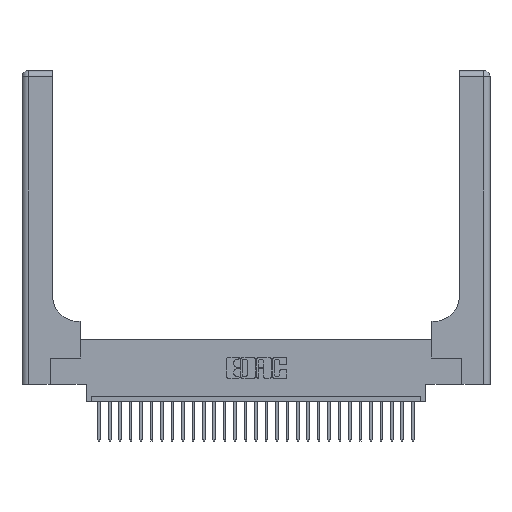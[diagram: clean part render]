
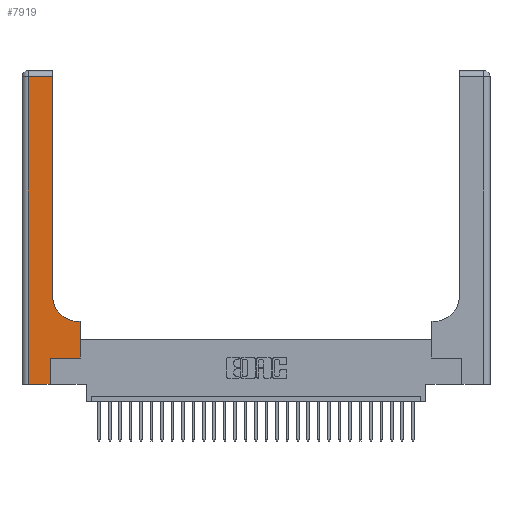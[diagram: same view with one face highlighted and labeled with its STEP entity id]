
A CAD part, top view. The second image highlights one B-rep face of the part: STEP entity #7919.
In plain terms, the highlighted planar face has unit normal (0, 0, 1).
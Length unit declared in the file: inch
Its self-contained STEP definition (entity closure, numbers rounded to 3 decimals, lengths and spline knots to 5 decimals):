
#313 = VECTOR ( 'NONE', #22695, 39.37008 ) ;
#1275 = LINE ( 'NONE', #13451, #19869 ) ;
#1321 = VERTEX_POINT ( 'NONE', #15081 ) ;
#1476 = VECTOR ( 'NONE', #20335, 39.37008 ) ;
#2177 = VERTEX_POINT ( 'NONE', #14005 ) ;
#2541 = VECTOR ( 'NONE', #29848, 39.37008 ) ;
#3033 = VERTEX_POINT ( 'NONE', #15591 ) ;
#3550 = LINE ( 'NONE', #24825, #9059 ) ;
#4838 = FACE_OUTER_BOUND ( 'NONE', #28960, .T. ) ;
#5357 = VERTEX_POINT ( 'NONE', #7960 ) ;
#5695 = CIRCLE ( 'NONE', #26918, 0.25 ) ;
#5790 = VECTOR ( 'NONE', #11148, 39.37008 ) ;
#6203 = VERTEX_POINT ( 'NONE', #27442 ) ;
#6899 = CARTESIAN_POINT ( 'NONE',  ( 0.5415, 0.85, 0.37 ) ) ;
#7050 = ORIENTED_EDGE ( 'NONE', *, *, #10753, .T. ) ;
#7227 = LINE ( 'NONE', #27291, #313 ) ;
#7815 = LINE ( 'NONE', #10754, #18358 ) ;
#7863 = DIRECTION ( 'NONE',  ( -1., 0., 0. ) ) ;
#7919 = ADVANCED_FACE ( 'NONE', ( #4838 ), #24490, .F. ) ;
#7934 = CARTESIAN_POINT ( 'NONE',  ( 0.269, 0.25, 0.37 ) ) ;
#7960 = CARTESIAN_POINT ( 'NONE',  ( 0.5585, 0.6, 0.37 ) ) ;
#8285 = CARTESIAN_POINT ( 'NONE',  ( 0., 3., 0.37 ) ) ;
#8692 = CARTESIAN_POINT ( 'NONE',  ( 0.06, 2.94, 0.37 ) ) ;
#9059 = VECTOR ( 'NONE', #10850, 39.37008 ) ;
#10523 = DIRECTION ( 'NONE',  ( 0., 0., -1. ) ) ;
#10753 = EDGE_CURVE ( 'NONE', #6203, #20432, #12018, .T. ) ;
#10754 = CARTESIAN_POINT ( 'NONE',  ( 0.2915, 0.6, 0.37 ) ) ;
#10850 = DIRECTION ( 'NONE',  ( 1., 0., 0. ) ) ;
#11148 = DIRECTION ( 'NONE',  ( -1., 0., 0. ) ) ;
#11509 = DIRECTION ( 'NONE',  ( 1., 0., 0. ) ) ;
#12018 = LINE ( 'NONE', #15990, #5790 ) ;
#12317 = EDGE_CURVE ( 'NONE', #16109, #14311, #1275, .T. ) ;
#12753 = ORIENTED_EDGE ( 'NONE', *, *, #21184, .T. ) ;
#13207 = CARTESIAN_POINT ( 'NONE',  ( 0.2915, 3., 0.37 ) ) ;
#13451 = CARTESIAN_POINT ( 'NONE',  ( 0.269, 0., 0.37 ) ) ;
#13736 = ORIENTED_EDGE ( 'NONE', *, *, #22083, .T. ) ;
#14005 = CARTESIAN_POINT ( 'NONE',  ( 0.5585, 0.25, 0.37 ) ) ;
#14012 = ORIENTED_EDGE ( 'NONE', *, *, #25195, .T. ) ;
#14311 = VERTEX_POINT ( 'NONE', #7934 ) ;
#14428 = ORIENTED_EDGE ( 'NONE', *, *, #27021, .T. ) ;
#15081 = CARTESIAN_POINT ( 'NONE',  ( 0.2915, 0.85, 0.37 ) ) ;
#15227 = ORIENTED_EDGE ( 'NONE', *, *, #12317, .T. ) ;
#15591 = CARTESIAN_POINT ( 'NONE',  ( 0.5415, 0.6, 0.37 ) ) ;
#15620 = ORIENTED_EDGE ( 'NONE', *, *, #22857, .T. ) ;
#15990 = CARTESIAN_POINT ( 'NONE',  ( 0., 2.94, 0.37 ) ) ;
#16078 = CARTESIAN_POINT ( 'NONE',  ( 0., 0., 0.37 ) ) ;
#16109 = VERTEX_POINT ( 'NONE', #17116 ) ;
#16749 = LINE ( 'NONE', #16078, #2541 ) ;
#17116 = CARTESIAN_POINT ( 'NONE',  ( 0.269, 0., 0.37 ) ) ;
#17166 = VERTEX_POINT ( 'NONE', #26874 ) ;
#17560 = DIRECTION ( 'NONE',  ( 0., 1., 0. ) ) ;
#17983 = AXIS2_PLACEMENT_3D ( 'NONE', #8285, #10523, #7863 ) ;
#18252 = DIRECTION ( 'NONE',  ( -1., 0., 0. ) ) ;
#18358 = VECTOR ( 'NONE', #18252, 39.37008 ) ;
#19869 = VECTOR ( 'NONE', #20549, 39.37008 ) ;
#20335 = DIRECTION ( 'NONE',  ( 0., 1., 0. ) ) ;
#20432 = VERTEX_POINT ( 'NONE', #8692 ) ;
#20549 = DIRECTION ( 'NONE',  ( 0., 1., 0. ) ) ;
#20609 = ORIENTED_EDGE ( 'NONE', *, *, #21494, .T. ) ;
#21184 = EDGE_CURVE ( 'NONE', #2177, #5357, #26303, .T. ) ;
#21494 = EDGE_CURVE ( 'NONE', #17166, #16109, #16749, .T. ) ;
#22083 = EDGE_CURVE ( 'NONE', #20432, #17166, #7227, .T. ) ;
#22695 = DIRECTION ( 'NONE',  ( 0., -1., 0. ) ) ;
#22815 = LINE ( 'NONE', #13207, #29333 ) ;
#22857 = EDGE_CURVE ( 'NONE', #14311, #2177, #3550, .T. ) ;
#23156 = ORIENTED_EDGE ( 'NONE', *, *, #23455, .T. ) ;
#23455 = EDGE_CURVE ( 'NONE', #3033, #1321, #5695, .T. ) ;
#24490 = PLANE ( 'NONE',  #17983 ) ;
#24664 = CARTESIAN_POINT ( 'NONE',  ( 0.5585, 0.25, 0.37 ) ) ;
#24825 = CARTESIAN_POINT ( 'NONE',  ( 0.269, 0.25, 0.37 ) ) ;
#25195 = EDGE_CURVE ( 'NONE', #1321, #6203, #22815, .T. ) ;
#26303 = LINE ( 'NONE', #24664, #1476 ) ;
#26874 = CARTESIAN_POINT ( 'NONE',  ( 0.06, 0., 0.37 ) ) ;
#26918 = AXIS2_PLACEMENT_3D ( 'NONE', #6899, #30027, #11509 ) ;
#27021 = EDGE_CURVE ( 'NONE', #5357, #3033, #7815, .T. ) ;
#27291 = CARTESIAN_POINT ( 'NONE',  ( 0.06, 3., 0.37 ) ) ;
#27442 = CARTESIAN_POINT ( 'NONE',  ( 0.2915, 2.94, 0.37 ) ) ;
#28960 = EDGE_LOOP ( 'NONE', ( #14012, #7050, #13736, #20609, #15227, #15620, #12753, #14428, #23156 ) ) ;
#29333 = VECTOR ( 'NONE', #17560, 39.37008 ) ;
#29848 = DIRECTION ( 'NONE',  ( 1., 0., 0. ) ) ;
#30027 = DIRECTION ( 'NONE',  ( 0., 0., -1. ) ) ;
